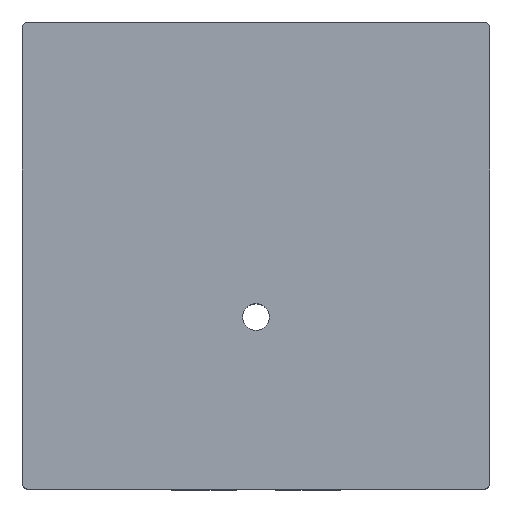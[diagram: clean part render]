
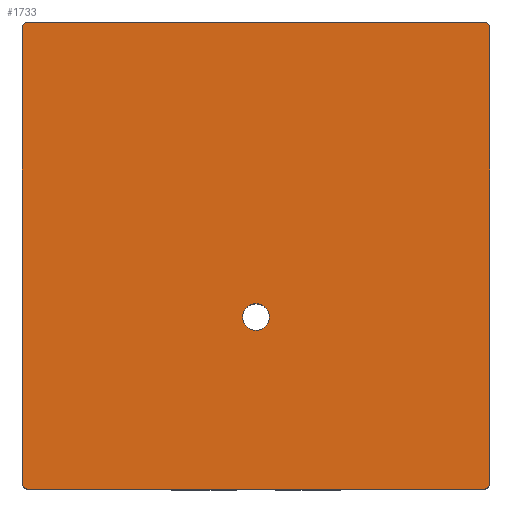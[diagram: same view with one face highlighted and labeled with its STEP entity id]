
A CAD part, top view. The second image highlights one B-rep face of the part: STEP entity #1733.
In plain terms, the highlighted planar face has unit normal (0, 0, 1).
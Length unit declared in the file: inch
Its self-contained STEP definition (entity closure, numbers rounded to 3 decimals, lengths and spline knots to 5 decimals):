
#99=LINE('',#2476,#244);
#178=LINE('',#2767,#323);
#225=LINE('',#3088,#370);
#226=LINE('',#3089,#371);
#244=VECTOR('',#1978,0.3937);
#323=VECTOR('',#2321,0.3937);
#370=VECTOR('',#2408,0.3937);
#371=VECTOR('',#2409,0.3937);
#399=PLANE('',#1925);
#409=FACE_BOUND('',#619,.T.);
#509=FACE_OUTER_BOUND('',#618,.T.);
#618=EDGE_LOOP('',(#1549,#1550,#1551,#1552,#1553,#1554,#1555,#1556));
#619=EDGE_LOOP('',(#1557));
#626=CIRCLE('',#1761,0.0575);
#650=CIRCLE('',#1808,0.025);
#685=CIRCLE('',#1873,0.025);
#686=CIRCLE('',#1884,0.025);
#687=CIRCLE('',#1890,0.025);
#693=VERTEX_POINT('',#2425);
#713=VERTEX_POINT('',#2473);
#714=VERTEX_POINT('',#2475);
#742=VERTEX_POINT('',#2557);
#780=VERTEX_POINT('',#2679);
#783=VERTEX_POINT('',#2709);
#784=VERTEX_POINT('',#2710);
#787=VERTEX_POINT('',#2727);
#788=VERTEX_POINT('',#2728);
#841=EDGE_CURVE('',#693,#693,#626,.T.);
#865=EDGE_CURVE('',#714,#713,#99,.T.);
#905=EDGE_CURVE('',#742,#713,#650,.T.);
#964=EDGE_CURVE('',#714,#780,#685,.T.);
#982=EDGE_CURVE('',#783,#784,#686,.T.);
#992=EDGE_CURVE('',#787,#788,#687,.T.);
#1014=EDGE_CURVE('',#742,#788,#178,.T.);
#1088=EDGE_CURVE('',#787,#784,#225,.T.);
#1089=EDGE_CURVE('',#783,#780,#226,.T.);
#1549=ORIENTED_EDGE('',*,*,#964,.F.);
#1550=ORIENTED_EDGE('',*,*,#865,.T.);
#1551=ORIENTED_EDGE('',*,*,#905,.F.);
#1552=ORIENTED_EDGE('',*,*,#1014,.T.);
#1553=ORIENTED_EDGE('',*,*,#992,.F.);
#1554=ORIENTED_EDGE('',*,*,#1088,.T.);
#1555=ORIENTED_EDGE('',*,*,#982,.F.);
#1556=ORIENTED_EDGE('',*,*,#1089,.T.);
#1557=ORIENTED_EDGE('',*,*,#841,.T.);
#1733=ADVANCED_FACE('',(#509,#409),#399,.T.);
#1761=AXIS2_PLACEMENT_3D('',#2426,#1936,#1937);
#1808=AXIS2_PLACEMENT_3D('',#2558,#2066,#2067);
#1873=AXIS2_PLACEMENT_3D('',#2680,#2215,#2216);
#1884=AXIS2_PLACEMENT_3D('',#2711,#2253,#2254);
#1890=AXIS2_PLACEMENT_3D('',#2729,#2273,#2274);
#1925=AXIS2_PLACEMENT_3D('',#3087,#2406,#2407);
#1936=DIRECTION('center_axis',(0.,0.,-1.));
#1937=DIRECTION('ref_axis',(1.,0.,0.));
#1978=DIRECTION('',(1.,0.,0.));
#2066=DIRECTION('center_axis',(0.,0.,-1.));
#2067=DIRECTION('ref_axis',(0.707,-0.707,0.));
#2215=DIRECTION('center_axis',(0.,0.,-1.));
#2216=DIRECTION('ref_axis',(-0.707,-0.707,0.));
#2253=DIRECTION('center_axis',(0.,0.,-1.));
#2254=DIRECTION('ref_axis',(-0.707,0.707,0.));
#2273=DIRECTION('center_axis',(0.,0.,-1.));
#2274=DIRECTION('ref_axis',(0.707,0.707,0.));
#2321=DIRECTION('',(0.,1.,0.));
#2406=DIRECTION('center_axis',(0.,0.,1.));
#2407=DIRECTION('ref_axis',(1.,0.,0.));
#2408=DIRECTION('',(-1.,0.,0.));
#2409=DIRECTION('',(0.,-1.,0.));
#2425=CARTESIAN_POINT('',(0.9425,0.73718,2.));
#2426=CARTESIAN_POINT('Origin',(1.,0.73718,2.));
#2473=CARTESIAN_POINT('',(1.975,0.,2.));
#2475=CARTESIAN_POINT('',(0.025,0.,2.));
#2476=CARTESIAN_POINT('',(0.,0.,2.));
#2557=CARTESIAN_POINT('',(2.,0.025,2.));
#2558=CARTESIAN_POINT('Origin',(1.975,0.025,2.));
#2679=CARTESIAN_POINT('',(0.,0.025,2.));
#2680=CARTESIAN_POINT('Origin',(0.025,0.025,2.));
#2709=CARTESIAN_POINT('',(0.,1.975,2.));
#2710=CARTESIAN_POINT('',(0.025,2.,2.));
#2711=CARTESIAN_POINT('Origin',(0.025,1.975,2.));
#2727=CARTESIAN_POINT('',(1.975,2.,2.));
#2728=CARTESIAN_POINT('',(2.,1.975,2.));
#2729=CARTESIAN_POINT('Origin',(1.975,1.975,2.));
#2767=CARTESIAN_POINT('',(2.,0.,2.));
#3087=CARTESIAN_POINT('Origin',(1.,1.,2.));
#3088=CARTESIAN_POINT('',(2.,2.,2.));
#3089=CARTESIAN_POINT('',(0.,2.,2.));
